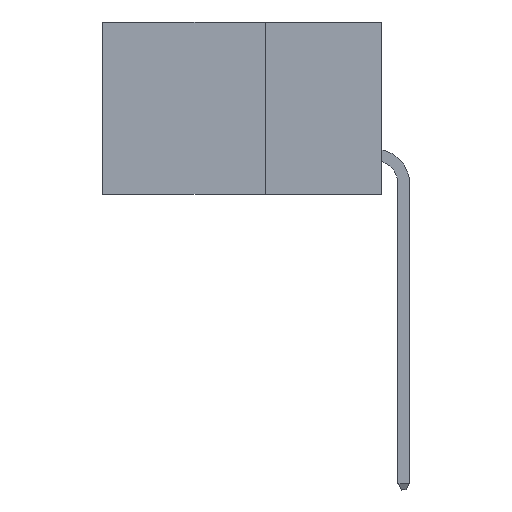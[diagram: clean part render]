
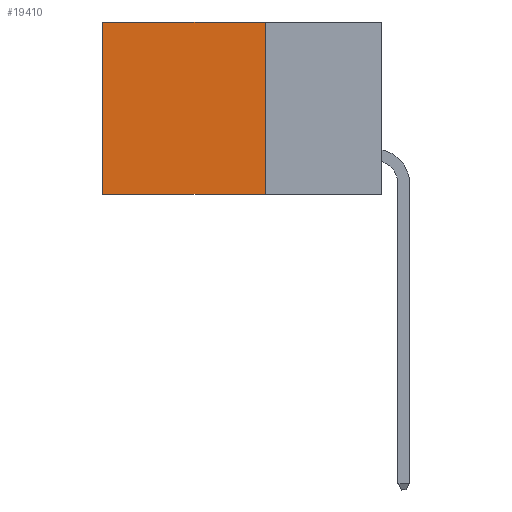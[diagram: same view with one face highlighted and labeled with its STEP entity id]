
A CAD part, left-side view. The second image highlights one B-rep face of the part: STEP entity #19410.
In plain terms, the highlighted planar face has unit normal (-1, 0, 0).
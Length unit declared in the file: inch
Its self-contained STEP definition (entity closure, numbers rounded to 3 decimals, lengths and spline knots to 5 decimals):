
#3242 = CARTESIAN_POINT ( 'NONE',  ( 0.2875, 0.25, 0. ) ) ;
#4335 = EDGE_CURVE ( 'NONE', #29463, #50802, #47746, .T. ) ;
#4728 = VECTOR ( 'NONE', #5665, 39.37008 ) ;
#5665 = DIRECTION ( 'NONE',  ( 0., 1., 0. ) ) ;
#5682 = DIRECTION ( 'NONE',  ( 0., 0., -1. ) ) ;
#6023 = CARTESIAN_POINT ( 'NONE',  ( 0.2875, 0.25, -0.37 ) ) ;
#9289 = EDGE_CURVE ( 'NONE', #42443, #29463, #26456, .T. ) ;
#13942 = CARTESIAN_POINT ( 'NONE',  ( 0.2875, 0.6, -0.37 ) ) ;
#15718 = EDGE_CURVE ( 'NONE', #42443, #28611, #20767, .T. ) ;
#17986 = ORIENTED_EDGE ( 'NONE', *, *, #4335, .T. ) ;
#18208 = CARTESIAN_POINT ( 'NONE',  ( 0.2875, 0.25, 0. ) ) ;
#18525 = CARTESIAN_POINT ( 'NONE',  ( 0.2875, 0.25, -0.37 ) ) ;
#19410 = ADVANCED_FACE ( 'NONE', ( #19810 ), #50343, .F. ) ;
#19810 = FACE_OUTER_BOUND ( 'NONE', #31631, .T. ) ;
#19929 = ORIENTED_EDGE ( 'NONE', *, *, #15718, .F. ) ;
#20767 = LINE ( 'NONE', #30003, #36844 ) ;
#21359 = CARTESIAN_POINT ( 'NONE',  ( 0.2875, 0.6, 0. ) ) ;
#21506 = ORIENTED_EDGE ( 'NONE', *, *, #9289, .T. ) ;
#22195 = LINE ( 'NONE', #6023, #4728 ) ;
#24210 = VECTOR ( 'NONE', #5682, 39.37008 ) ;
#25539 = AXIS2_PLACEMENT_3D ( 'NONE', #39082, #26578, #42551 ) ;
#26456 = LINE ( 'NONE', #3242, #34531 ) ;
#26578 = DIRECTION ( 'NONE',  ( 1., 0., 0. ) ) ;
#28611 = VERTEX_POINT ( 'NONE', #18525 ) ;
#29463 = VERTEX_POINT ( 'NONE', #37885 ) ;
#30003 = CARTESIAN_POINT ( 'NONE',  ( 0.2875, 0.25, 0. ) ) ;
#30947 = ORIENTED_EDGE ( 'NONE', *, *, #40085, .F. ) ;
#31631 = EDGE_LOOP ( 'NONE', ( #17986, #30947, #19929, #21506 ) ) ;
#34531 = VECTOR ( 'NONE', #39198, 39.37008 ) ;
#36844 = VECTOR ( 'NONE', #43972, 39.37008 ) ;
#37885 = CARTESIAN_POINT ( 'NONE',  ( 0.2875, 0.6, 0. ) ) ;
#39082 = CARTESIAN_POINT ( 'NONE',  ( 0.2875, 0.25, 0. ) ) ;
#39198 = DIRECTION ( 'NONE',  ( 0., 1., 0. ) ) ;
#40085 = EDGE_CURVE ( 'NONE', #28611, #50802, #22195, .T. ) ;
#42443 = VERTEX_POINT ( 'NONE', #18208 ) ;
#42551 = DIRECTION ( 'NONE',  ( 0., 0., -1. ) ) ;
#43972 = DIRECTION ( 'NONE',  ( 0., 0., -1. ) ) ;
#47746 = LINE ( 'NONE', #21359, #24210 ) ;
#50343 = PLANE ( 'NONE',  #25539 ) ;
#50802 = VERTEX_POINT ( 'NONE', #13942 ) ;
